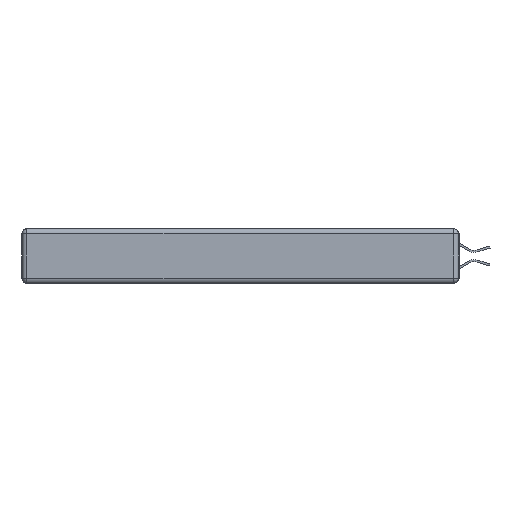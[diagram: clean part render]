
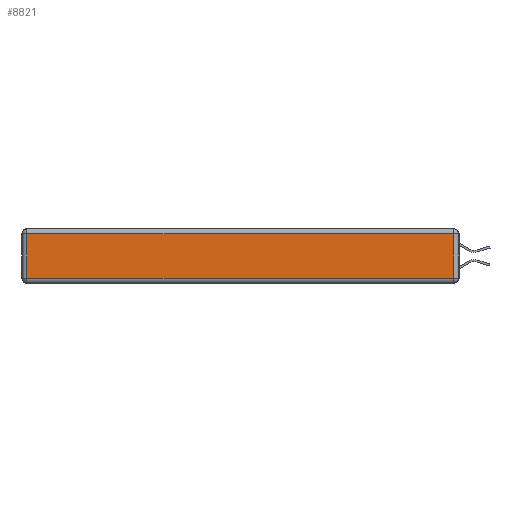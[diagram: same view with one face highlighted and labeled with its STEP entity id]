
A CAD part, left-side view. The second image highlights one B-rep face of the part: STEP entity #8821.
In plain terms, the highlighted planar face has unit normal (-1, 0, 0).
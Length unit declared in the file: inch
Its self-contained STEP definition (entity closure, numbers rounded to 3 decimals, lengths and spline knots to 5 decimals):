
#967 = DIRECTION ( 'NONE',  ( 0., 0., 1. ) ) ;
#1662 = VERTEX_POINT ( 'NONE', #2202 ) ;
#1854 = CARTESIAN_POINT ( 'NONE',  ( 0., 0.03, -0.313 ) ) ;
#1958 = CARTESIAN_POINT ( 'NONE',  ( 0., 2.72, -0.343 ) ) ;
#2202 = CARTESIAN_POINT ( 'NONE',  ( 0., 2.72, -0.03 ) ) ;
#3134 = LINE ( 'NONE', #1958, #16565 ) ;
#3539 = DIRECTION ( 'NONE',  ( 0., 0., -1. ) ) ;
#4137 = VECTOR ( 'NONE', #9786, 39.37008 ) ;
#4247 = VECTOR ( 'NONE', #19209, 39.37008 ) ;
#7368 = AXIS2_PLACEMENT_3D ( 'NONE', #8726, #11754, #967 ) ;
#8518 = CARTESIAN_POINT ( 'NONE',  ( 0., 0.03, -0.343 ) ) ;
#8726 = CARTESIAN_POINT ( 'NONE',  ( 0., 0., -0.343 ) ) ;
#8821 = ADVANCED_FACE ( 'NONE', ( #17979 ), #16457, .T. ) ;
#9786 = DIRECTION ( 'NONE',  ( 0., 1., 0. ) ) ;
#10355 = CARTESIAN_POINT ( 'NONE',  ( 0., 2.72, -0.313 ) ) ;
#10765 = CARTESIAN_POINT ( 'NONE',  ( 0., 0.03, -0.03 ) ) ;
#10811 = LINE ( 'NONE', #8518, #4247 ) ;
#11388 = VECTOR ( 'NONE', #17023, 39.37008 ) ;
#11429 = LINE ( 'NONE', #14578, #4137 ) ;
#11754 = DIRECTION ( 'NONE',  ( -1., 0., 0. ) ) ;
#11760 = VERTEX_POINT ( 'NONE', #1854 ) ;
#14081 = LINE ( 'NONE', #15579, #11388 ) ;
#14550 = ORIENTED_EDGE ( 'NONE', *, *, #15675, .T. ) ;
#14578 = CARTESIAN_POINT ( 'NONE',  ( 0., 2.75, -0.03 ) ) ;
#15169 = EDGE_CURVE ( 'NONE', #1662, #19759, #3134, .T. ) ;
#15579 = CARTESIAN_POINT ( 'NONE',  ( 0., 0., -0.313 ) ) ;
#15675 = EDGE_CURVE ( 'NONE', #19759, #11760, #14081, .T. ) ;
#16457 = PLANE ( 'NONE',  #7368 ) ;
#16565 = VECTOR ( 'NONE', #3539, 39.37008 ) ;
#17023 = DIRECTION ( 'NONE',  ( 0., -1., 0. ) ) ;
#17184 = ORIENTED_EDGE ( 'NONE', *, *, #20138, .T. ) ;
#17419 = EDGE_CURVE ( 'NONE', #11760, #19318, #10811, .T. ) ;
#17979 = FACE_OUTER_BOUND ( 'NONE', #20275, .T. ) ;
#18648 = ORIENTED_EDGE ( 'NONE', *, *, #15169, .T. ) ;
#19209 = DIRECTION ( 'NONE',  ( 0., 0., 1. ) ) ;
#19318 = VERTEX_POINT ( 'NONE', #10765 ) ;
#19587 = ORIENTED_EDGE ( 'NONE', *, *, #17419, .T. ) ;
#19759 = VERTEX_POINT ( 'NONE', #10355 ) ;
#20138 = EDGE_CURVE ( 'NONE', #19318, #1662, #11429, .T. ) ;
#20275 = EDGE_LOOP ( 'NONE', ( #14550, #19587, #17184, #18648 ) ) ;
